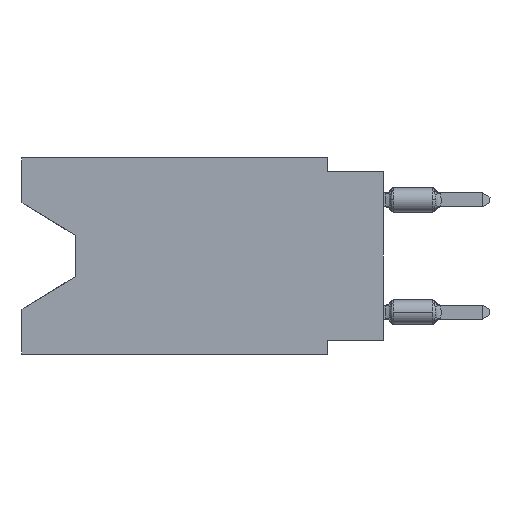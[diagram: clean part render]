
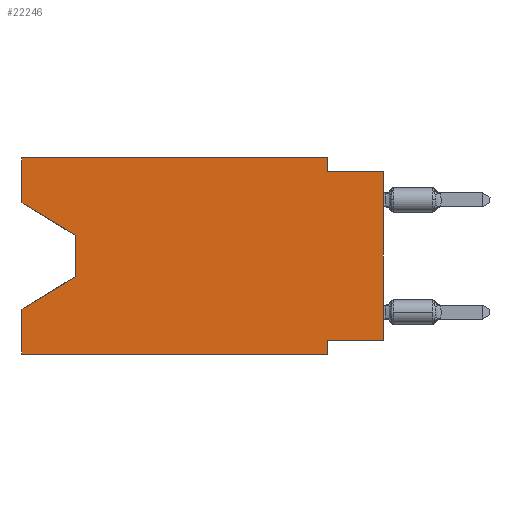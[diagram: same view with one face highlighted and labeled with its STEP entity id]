
A CAD part, left-side view. The second image highlights one B-rep face of the part: STEP entity #22246.
In plain terms, the highlighted planar face has unit normal (-1, 0, 0).
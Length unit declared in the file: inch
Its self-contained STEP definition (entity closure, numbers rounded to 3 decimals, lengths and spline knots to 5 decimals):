
#155 = CARTESIAN_POINT ( 'NONE',  ( 0., 0.55, -0.138 ) ) ;
#174 = DIRECTION ( 'NONE',  ( 0., -0.855, -0.519 ) ) ;
#194 = LINE ( 'NONE', #21760, #12365 ) ;
#319 = DIRECTION ( 'NONE',  ( 0., 0., 1. ) ) ;
#412 = VECTOR ( 'NONE', #24668, 39.37008 ) ;
#485 = LINE ( 'NONE', #9487, #13636 ) ;
#698 = CARTESIAN_POINT ( 'NONE',  ( 0., 0.645, 0. ) ) ;
#828 = VECTOR ( 'NONE', #14662, 39.37008 ) ;
#1210 = VECTOR ( 'NONE', #319, 39.37008 ) ;
#1259 = EDGE_CURVE ( 'NONE', #8578, #9662, #17451, .T. ) ;
#1563 = LINE ( 'NONE', #20445, #20872 ) ;
#1926 = CARTESIAN_POINT ( 'NONE',  ( 0., 0.1, 0. ) ) ;
#2041 = LINE ( 'NONE', #19295, #22181 ) ;
#2223 = FACE_OUTER_BOUND ( 'NONE', #10444, .T. ) ;
#2339 = EDGE_CURVE ( 'NONE', #13400, #9662, #1563, .T. ) ;
#2747 = CARTESIAN_POINT ( 'NONE',  ( 0., 0., -0.325 ) ) ;
#2787 = VECTOR ( 'NONE', #17770, 39.37008 ) ;
#2977 = EDGE_CURVE ( 'NONE', #10695, #9658, #2041, .T. ) ;
#3650 = CARTESIAN_POINT ( 'NONE',  ( 0., 0.1, 0. ) ) ;
#3851 = CARTESIAN_POINT ( 'NONE',  ( 0., 0.645, 0. ) ) ;
#4133 = VERTEX_POINT ( 'NONE', #21509 ) ;
#4314 = PLANE ( 'NONE',  #16453 ) ;
#4504 = DIRECTION ( 'NONE',  ( 0., 0.855, -0.519 ) ) ;
#4773 = CARTESIAN_POINT ( 'NONE',  ( 0., 0.645, -0.35 ) ) ;
#5709 = VECTOR ( 'NONE', #14538, 39.37008 ) ;
#5884 = ORIENTED_EDGE ( 'NONE', *, *, #21578, .T. ) ;
#5885 = ORIENTED_EDGE ( 'NONE', *, *, #16936, .T. ) ;
#7133 = EDGE_CURVE ( 'NONE', #10374, #22920, #8372, .T. ) ;
#7585 = LINE ( 'NONE', #3851, #9179 ) ;
#7932 = CARTESIAN_POINT ( 'NONE',  ( 0., 0.645, -0.26975 ) ) ;
#8107 = DIRECTION ( 'NONE',  ( 0., 0., -1. ) ) ;
#8372 = LINE ( 'NONE', #10243, #19625 ) ;
#8408 = CARTESIAN_POINT ( 'NONE',  ( 0., 0.1, -0.025 ) ) ;
#8542 = ORIENTED_EDGE ( 'NONE', *, *, #19215, .F. ) ;
#8578 = VERTEX_POINT ( 'NONE', #9005 ) ;
#9005 = CARTESIAN_POINT ( 'NONE',  ( 0., 0., -0.325 ) ) ;
#9035 = ORIENTED_EDGE ( 'NONE', *, *, #18257, .F. ) ;
#9179 = VECTOR ( 'NONE', #18854, 39.37008 ) ;
#9487 = CARTESIAN_POINT ( 'NONE',  ( 0., 0.1, -0.35 ) ) ;
#9658 = VERTEX_POINT ( 'NONE', #16007 ) ;
#9662 = VERTEX_POINT ( 'NONE', #19319 ) ;
#10243 = CARTESIAN_POINT ( 'NONE',  ( 0., 0.55, -0.212 ) ) ;
#10374 = VERTEX_POINT ( 'NONE', #23087 ) ;
#10383 = EDGE_CURVE ( 'NONE', #21439, #21250, #7585, .T. ) ;
#10444 = EDGE_LOOP ( 'NONE', ( #21026, #5885, #17208, #11574, #5884, #12330, #17038, #13039, #20463, #8542, #17141, #9035 ) ) ;
#10695 = VERTEX_POINT ( 'NONE', #20196 ) ;
#10972 = CARTESIAN_POINT ( 'NONE',  ( 0., 0.1, -0.325 ) ) ;
#11188 = DIRECTION ( 'NONE',  ( 0., -1., 0. ) ) ;
#11574 = ORIENTED_EDGE ( 'NONE', *, *, #18864, .F. ) ;
#12076 = DIRECTION ( 'NONE',  ( 0., 0., -1. ) ) ;
#12330 = ORIENTED_EDGE ( 'NONE', *, *, #19811, .F. ) ;
#12365 = VECTOR ( 'NONE', #21876, 39.37008 ) ;
#13039 = ORIENTED_EDGE ( 'NONE', *, *, #1259, .T. ) ;
#13082 = VERTEX_POINT ( 'NONE', #20945 ) ;
#13138 = VECTOR ( 'NONE', #21028, 39.37008 ) ;
#13400 = VERTEX_POINT ( 'NONE', #8408 ) ;
#13636 = VECTOR ( 'NONE', #8107, 39.37008 ) ;
#14309 = VERTEX_POINT ( 'NONE', #10972 ) ;
#14538 = DIRECTION ( 'NONE',  ( 0., -1., 0. ) ) ;
#14662 = DIRECTION ( 'NONE',  ( 0., 0., -1. ) ) ;
#14808 = CARTESIAN_POINT ( 'NONE',  ( 0., 0.645, 0. ) ) ;
#16007 = CARTESIAN_POINT ( 'NONE',  ( 0., 0.55, -0.138 ) ) ;
#16453 = AXIS2_PLACEMENT_3D ( 'NONE', #698, #17707, #12076 ) ;
#16936 = EDGE_CURVE ( 'NONE', #9658, #10374, #17150, .T. ) ;
#17038 = ORIENTED_EDGE ( 'NONE', *, *, #18168, .F. ) ;
#17067 = LINE ( 'NONE', #14808, #412 ) ;
#17141 = ORIENTED_EDGE ( 'NONE', *, *, #10383, .F. ) ;
#17150 = LINE ( 'NONE', #155, #13138 ) ;
#17208 = ORIENTED_EDGE ( 'NONE', *, *, #7133, .T. ) ;
#17451 = LINE ( 'NONE', #18824, #1210 ) ;
#17707 = DIRECTION ( 'NONE',  ( 1., 0., 0. ) ) ;
#17770 = DIRECTION ( 'NONE',  ( 0., 1., 0. ) ) ;
#18168 = EDGE_CURVE ( 'NONE', #8578, #14309, #22678, .T. ) ;
#18257 = EDGE_CURVE ( 'NONE', #10695, #21439, #194, .T. ) ;
#18824 = CARTESIAN_POINT ( 'NONE',  ( 0., 0., 0. ) ) ;
#18854 = DIRECTION ( 'NONE',  ( 0., -1., 0. ) ) ;
#18864 = EDGE_CURVE ( 'NONE', #13082, #22920, #17067, .T. ) ;
#19215 = EDGE_CURVE ( 'NONE', #21250, #13400, #20529, .T. ) ;
#19295 = CARTESIAN_POINT ( 'NONE',  ( 0., 0.645, -0.08025 ) ) ;
#19319 = CARTESIAN_POINT ( 'NONE',  ( 0., 0., -0.025 ) ) ;
#19431 = CARTESIAN_POINT ( 'NONE',  ( 0., 0.645, 0. ) ) ;
#19625 = VECTOR ( 'NONE', #4504, 39.37008 ) ;
#19811 = EDGE_CURVE ( 'NONE', #14309, #4133, #485, .T. ) ;
#20196 = CARTESIAN_POINT ( 'NONE',  ( 0., 0.645, -0.08025 ) ) ;
#20445 = CARTESIAN_POINT ( 'NONE',  ( 0., 0., -0.025 ) ) ;
#20463 = ORIENTED_EDGE ( 'NONE', *, *, #2339, .F. ) ;
#20529 = LINE ( 'NONE', #3650, #828 ) ;
#20872 = VECTOR ( 'NONE', #11188, 39.37008 ) ;
#20945 = CARTESIAN_POINT ( 'NONE',  ( 0., 0.645, -0.35 ) ) ;
#21026 = ORIENTED_EDGE ( 'NONE', *, *, #2977, .T. ) ;
#21028 = DIRECTION ( 'NONE',  ( 0., 0., -1. ) ) ;
#21250 = VERTEX_POINT ( 'NONE', #1926 ) ;
#21439 = VERTEX_POINT ( 'NONE', #19431 ) ;
#21509 = CARTESIAN_POINT ( 'NONE',  ( 0., 0.1, -0.35 ) ) ;
#21578 = EDGE_CURVE ( 'NONE', #13082, #4133, #23891, .T. ) ;
#21760 = CARTESIAN_POINT ( 'NONE',  ( 0., 0.645, 0. ) ) ;
#21876 = DIRECTION ( 'NONE',  ( 0., 0., 1. ) ) ;
#22181 = VECTOR ( 'NONE', #174, 39.37008 ) ;
#22246 = ADVANCED_FACE ( 'NONE', ( #2223 ), #4314, .F. ) ;
#22678 = LINE ( 'NONE', #2747, #2787 ) ;
#22920 = VERTEX_POINT ( 'NONE', #7932 ) ;
#23087 = CARTESIAN_POINT ( 'NONE',  ( 0., 0.55, -0.212 ) ) ;
#23891 = LINE ( 'NONE', #4773, #5709 ) ;
#24668 = DIRECTION ( 'NONE',  ( 0., 0., 1. ) ) ;
